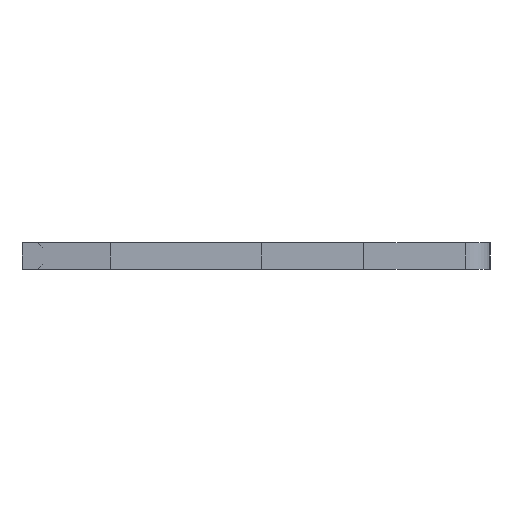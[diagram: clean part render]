
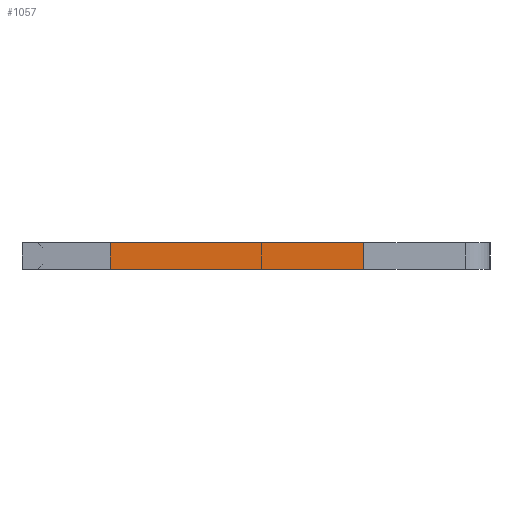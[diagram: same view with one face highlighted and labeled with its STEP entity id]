
A CAD part, left-side view. The second image highlights one B-rep face of the part: STEP entity #1057.
In plain terms, the highlighted face is planar.
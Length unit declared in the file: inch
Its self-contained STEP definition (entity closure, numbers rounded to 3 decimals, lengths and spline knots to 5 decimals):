
#224 = CARTESIAN_POINT ( 'NONE',  ( 0.013, 0.146, -0.0575 ) ) ;
#298 = VECTOR ( 'NONE', #2423, 39.37008 ) ;
#489 = CARTESIAN_POINT ( 'NONE',  ( 0.013, -0.099, -0.0575 ) ) ;
#533 = DIRECTION ( 'NONE',  ( -1., 0., 0. ) ) ;
#538 = EDGE_CURVE ( 'NONE', #1386, #980, #2375, .T. ) ;
#582 = ORIENTED_EDGE ( 'NONE', *, *, #677, .T. ) ;
#603 = VECTOR ( 'NONE', #533, 39.37008 ) ;
#648 = CARTESIAN_POINT ( 'NONE',  ( 0.013, -0.099, -0.0575 ) ) ;
#673 = VECTOR ( 'NONE', #969, 39.37008 ) ;
#677 = EDGE_CURVE ( 'NONE', #1749, #1386, #2612, .T. ) ;
#906 = LINE ( 'NONE', #2037, #673 ) ;
#920 = CARTESIAN_POINT ( 'NONE',  ( -0.013, 0.146, -0.0575 ) ) ;
#969 = DIRECTION ( 'NONE',  ( 0., 1., 0. ) ) ;
#974 = EDGE_LOOP ( 'NONE', ( #1888, #1751, #1517, #582 ) ) ;
#980 = VERTEX_POINT ( 'NONE', #2012 ) ;
#1023 = DIRECTION ( 'NONE',  ( 1., 0., 0. ) ) ;
#1052 = CARTESIAN_POINT ( 'NONE',  ( -0.013, -0.099, -0.0575 ) ) ;
#1057 = ADVANCED_FACE ( 'NONE', ( #2076 ), #1245, .F. ) ;
#1194 = CARTESIAN_POINT ( 'NONE',  ( 0.013, 0.146, -0.0575 ) ) ;
#1206 = VECTOR ( 'NONE', #2204, 39.37008 ) ;
#1245 = PLANE ( 'NONE',  #2229 ) ;
#1265 = DIRECTION ( 'NONE',  ( 0., 0., 1. ) ) ;
#1386 = VERTEX_POINT ( 'NONE', #1052 ) ;
#1517 = ORIENTED_EDGE ( 'NONE', *, *, #2482, .F. ) ;
#1749 = VERTEX_POINT ( 'NONE', #648 ) ;
#1751 = ORIENTED_EDGE ( 'NONE', *, *, #2393, .F. ) ;
#1888 = ORIENTED_EDGE ( 'NONE', *, *, #538, .T. ) ;
#1921 = VERTEX_POINT ( 'NONE', #2141 ) ;
#2012 = CARTESIAN_POINT ( 'NONE',  ( -0.013, 0.146, -0.0575 ) ) ;
#2037 = CARTESIAN_POINT ( 'NONE',  ( 0.013, 0.146, -0.0575 ) ) ;
#2076 = FACE_OUTER_BOUND ( 'NONE', #974, .T. ) ;
#2141 = CARTESIAN_POINT ( 'NONE',  ( 0.013, 0.146, -0.0575 ) ) ;
#2204 = DIRECTION ( 'NONE',  ( 0., 1., 0. ) ) ;
#2229 = AXIS2_PLACEMENT_3D ( 'NONE', #224, #1265, #1023 ) ;
#2375 = LINE ( 'NONE', #920, #1206 ) ;
#2393 = EDGE_CURVE ( 'NONE', #1921, #980, #2537, .T. ) ;
#2423 = DIRECTION ( 'NONE',  ( -1., 0., 0. ) ) ;
#2482 = EDGE_CURVE ( 'NONE', #1749, #1921, #906, .T. ) ;
#2537 = LINE ( 'NONE', #1194, #603 ) ;
#2612 = LINE ( 'NONE', #489, #298 ) ;
